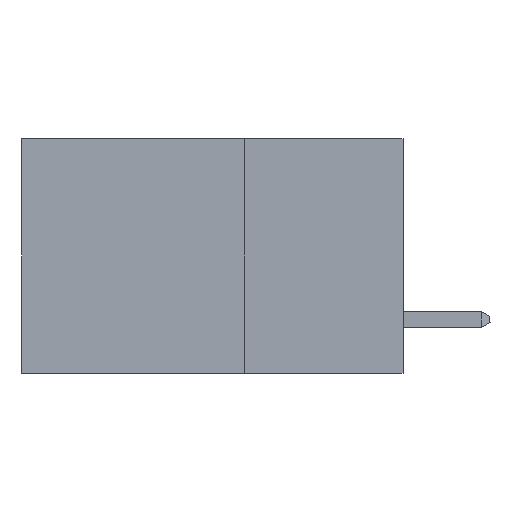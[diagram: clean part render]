
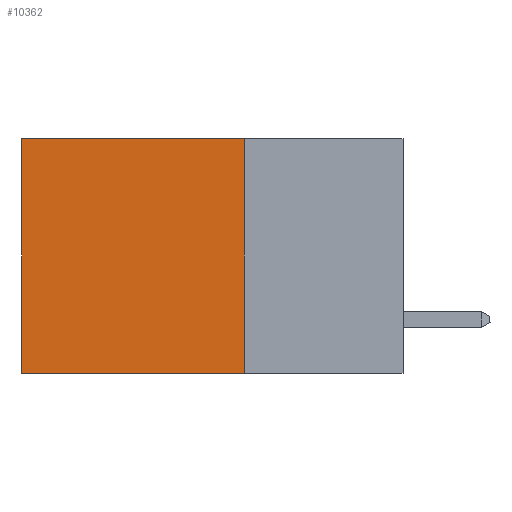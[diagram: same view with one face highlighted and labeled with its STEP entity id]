
A CAD part, left-side view. The second image highlights one B-rep face of the part: STEP entity #10362.
In plain terms, the highlighted planar face has unit normal (-1, 0, 0).
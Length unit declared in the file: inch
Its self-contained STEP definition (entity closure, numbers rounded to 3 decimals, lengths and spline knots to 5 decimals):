
#632 = ORIENTED_EDGE ( 'NONE', *, *, #6322, .T. ) ;
#1251 = CARTESIAN_POINT ( 'NONE',  ( 0.2875, 0.25, -0.37 ) ) ;
#1568 = CARTESIAN_POINT ( 'NONE',  ( 0.2875, 0.6, -0.37 ) ) ;
#2111 = DIRECTION ( 'NONE',  ( 0., 0., -1. ) ) ;
#3619 = VECTOR ( 'NONE', #2111, 39.37008 ) ;
#3827 = EDGE_CURVE ( 'NONE', #16242, #15718, #13350, .T. ) ;
#4531 = DIRECTION ( 'NONE',  ( 0., 1., 0. ) ) ;
#4775 = EDGE_LOOP ( 'NONE', ( #17209, #11902, #7386, #632 ) ) ;
#5201 = CARTESIAN_POINT ( 'NONE',  ( 0.2875, 0.6, 0. ) ) ;
#5456 = CARTESIAN_POINT ( 'NONE',  ( 0.2875, 0.25, 0. ) ) ;
#5618 = FACE_OUTER_BOUND ( 'NONE', #4775, .T. ) ;
#5731 = VERTEX_POINT ( 'NONE', #1568 ) ;
#6039 = CARTESIAN_POINT ( 'NONE',  ( 0.2875, 0.25, 0. ) ) ;
#6322 = EDGE_CURVE ( 'NONE', #16242, #12366, #7408, .T. ) ;
#6591 = DIRECTION ( 'NONE',  ( 1., 0., 0. ) ) ;
#7095 = CARTESIAN_POINT ( 'NONE',  ( 0.2875, 0.25, -0.37 ) ) ;
#7386 = ORIENTED_EDGE ( 'NONE', *, *, #3827, .F. ) ;
#7408 = LINE ( 'NONE', #6039, #16696 ) ;
#7677 = CARTESIAN_POINT ( 'NONE',  ( 0.2875, 0.25, 0. ) ) ;
#7913 = PLANE ( 'NONE',  #15731 ) ;
#8197 = EDGE_CURVE ( 'NONE', #15718, #5731, #9642, .T. ) ;
#9642 = LINE ( 'NONE', #1251, #16615 ) ;
#10362 = ADVANCED_FACE ( 'NONE', ( #5618 ), #7913, .F. ) ;
#10646 = DIRECTION ( 'NONE',  ( 0., 1., 0. ) ) ;
#11772 = DIRECTION ( 'NONE',  ( 0., 0., -1. ) ) ;
#11902 = ORIENTED_EDGE ( 'NONE', *, *, #8197, .F. ) ;
#12104 = VECTOR ( 'NONE', #15801, 39.37008 ) ;
#12366 = VERTEX_POINT ( 'NONE', #5201 ) ;
#12772 = CARTESIAN_POINT ( 'NONE',  ( 0.2875, 0.6, 0. ) ) ;
#13029 = CARTESIAN_POINT ( 'NONE',  ( 0.2875, 0.25, 0. ) ) ;
#13037 = LINE ( 'NONE', #12772, #3619 ) ;
#13350 = LINE ( 'NONE', #13029, #12104 ) ;
#15410 = EDGE_CURVE ( 'NONE', #12366, #5731, #13037, .T. ) ;
#15718 = VERTEX_POINT ( 'NONE', #7095 ) ;
#15731 = AXIS2_PLACEMENT_3D ( 'NONE', #7677, #6591, #11772 ) ;
#15801 = DIRECTION ( 'NONE',  ( 0., 0., -1. ) ) ;
#16242 = VERTEX_POINT ( 'NONE', #5456 ) ;
#16615 = VECTOR ( 'NONE', #10646, 39.37008 ) ;
#16696 = VECTOR ( 'NONE', #4531, 39.37008 ) ;
#17209 = ORIENTED_EDGE ( 'NONE', *, *, #15410, .T. ) ;
